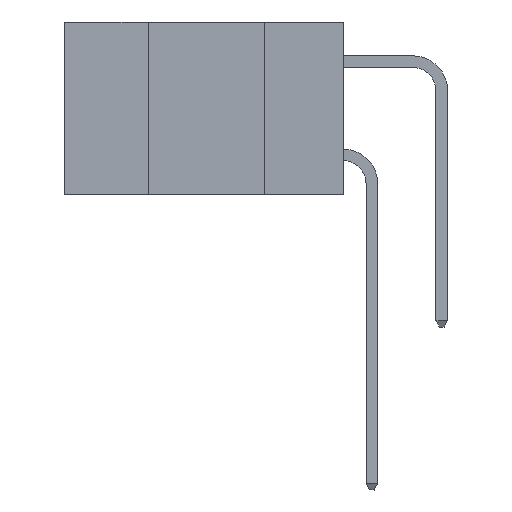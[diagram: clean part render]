
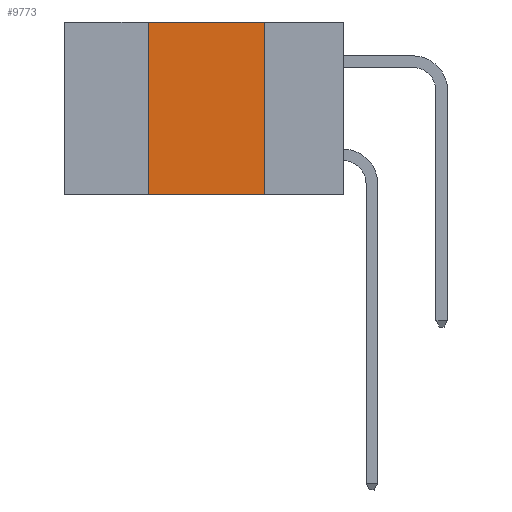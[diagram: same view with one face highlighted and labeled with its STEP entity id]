
A CAD part, left-side view. The second image highlights one B-rep face of the part: STEP entity #9773.
In plain terms, the highlighted planar face has unit normal (-1, 0, 0).
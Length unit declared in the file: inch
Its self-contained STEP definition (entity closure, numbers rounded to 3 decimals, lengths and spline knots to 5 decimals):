
#94 = DIRECTION ( 'NONE',  ( 0., 0., -1. ) ) ;
#138 = CARTESIAN_POINT ( 'NONE',  ( 0., 0.6, -0.37 ) ) ;
#335 = FACE_OUTER_BOUND ( 'NONE', #17049, .T. ) ;
#1124 = EDGE_CURVE ( 'NONE', #12928, #5758, #18328, .T. ) ;
#2288 = CARTESIAN_POINT ( 'NONE',  ( 0., 0.17, -0.37 ) ) ;
#2599 = VECTOR ( 'NONE', #17323, 39.37008 ) ;
#2916 = VERTEX_POINT ( 'NONE', #12715 ) ;
#4481 = CARTESIAN_POINT ( 'NONE',  ( 0., 0.42, -0.37 ) ) ;
#4717 = PLANE ( 'NONE',  #16794 ) ;
#5099 = CARTESIAN_POINT ( 'NONE',  ( 0., 0.42, -0.37 ) ) ;
#5758 = VERTEX_POINT ( 'NONE', #2288 ) ;
#6012 = ORIENTED_EDGE ( 'NONE', *, *, #8024, .F. ) ;
#6524 = VECTOR ( 'NONE', #15828, 39.37008 ) ;
#6603 = ORIENTED_EDGE ( 'NONE', *, *, #1124, .F. ) ;
#6969 = ORIENTED_EDGE ( 'NONE', *, *, #16058, .T. ) ;
#8024 = EDGE_CURVE ( 'NONE', #10170, #2916, #10192, .T. ) ;
#9591 = DIRECTION ( 'NONE',  ( 0., 0., -1. ) ) ;
#9773 = ADVANCED_FACE ( 'NONE', ( #335 ), #4717, .F. ) ;
#9860 = VECTOR ( 'NONE', #9591, 39.37008 ) ;
#10170 = VERTEX_POINT ( 'NONE', #4481 ) ;
#10192 = LINE ( 'NONE', #5099, #2599 ) ;
#11459 = DIRECTION ( 'NONE',  ( 0., -1., 0. ) ) ;
#11711 = CARTESIAN_POINT ( 'NONE',  ( 0., 0.17, 0. ) ) ;
#12715 = CARTESIAN_POINT ( 'NONE',  ( 0., 0.42, 0. ) ) ;
#12928 = VERTEX_POINT ( 'NONE', #11711 ) ;
#15770 = ORIENTED_EDGE ( 'NONE', *, *, #22586, .F. ) ;
#15828 = DIRECTION ( 'NONE',  ( 0., -1., 0. ) ) ;
#16058 = EDGE_CURVE ( 'NONE', #10170, #5758, #17585, .T. ) ;
#16718 = CARTESIAN_POINT ( 'NONE',  ( 0., 0.6, 0. ) ) ;
#16794 = AXIS2_PLACEMENT_3D ( 'NONE', #17649, #19382, #94 ) ;
#17049 = EDGE_LOOP ( 'NONE', ( #6603, #15770, #6012, #6969 ) ) ;
#17323 = DIRECTION ( 'NONE',  ( 0., 0., 1. ) ) ;
#17585 = LINE ( 'NONE', #138, #6524 ) ;
#17649 = CARTESIAN_POINT ( 'NONE',  ( 0., 0.6, 0. ) ) ;
#18328 = LINE ( 'NONE', #21831, #9860 ) ;
#19382 = DIRECTION ( 'NONE',  ( 1., 0., 0. ) ) ;
#20424 = LINE ( 'NONE', #16718, #22852 ) ;
#21831 = CARTESIAN_POINT ( 'NONE',  ( 0., 0.17, -0.37 ) ) ;
#22586 = EDGE_CURVE ( 'NONE', #2916, #12928, #20424, .T. ) ;
#22852 = VECTOR ( 'NONE', #11459, 39.37008 ) ;
